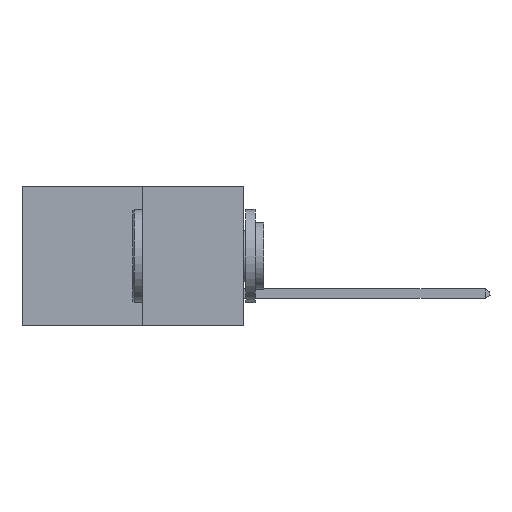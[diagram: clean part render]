
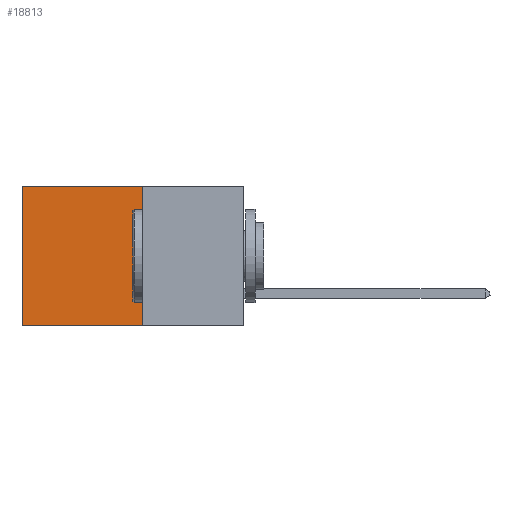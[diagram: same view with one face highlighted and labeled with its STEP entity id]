
A CAD part, left-side view. The second image highlights one B-rep face of the part: STEP entity #18813.
In plain terms, the highlighted planar face has unit normal (-1, 0, 0).
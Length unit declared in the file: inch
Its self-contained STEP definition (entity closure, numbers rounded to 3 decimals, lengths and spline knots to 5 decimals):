
#637 = ORIENTED_EDGE ( 'NONE', *, *, #9866, .T. ) ;
#1463 = LINE ( 'NONE', #20418, #7314 ) ;
#3775 = EDGE_LOOP ( 'NONE', ( #637, #26534, #28555, #9381 ) ) ;
#4281 = LINE ( 'NONE', #24166, #23272 ) ;
#5421 = CARTESIAN_POINT ( 'NONE',  ( 0.277, 0.59, -0.37 ) ) ;
#5788 = EDGE_CURVE ( 'NONE', #28523, #26337, #24713, .T. ) ;
#7314 = VECTOR ( 'NONE', #10616, 39.37008 ) ;
#8589 = CARTESIAN_POINT ( 'NONE',  ( 0.277, 0.27, -0.37 ) ) ;
#8829 = VERTEX_POINT ( 'NONE', #9032 ) ;
#9032 = CARTESIAN_POINT ( 'NONE',  ( 0.277, 0.59, 0. ) ) ;
#9381 = ORIENTED_EDGE ( 'NONE', *, *, #26235, .T. ) ;
#9478 = FACE_OUTER_BOUND ( 'NONE', #3775, .T. ) ;
#9866 = EDGE_CURVE ( 'NONE', #8829, #26337, #4281, .T. ) ;
#10616 = DIRECTION ( 'NONE',  ( 0., 0., -1. ) ) ;
#11100 = DIRECTION ( 'NONE',  ( 0., 0., -1. ) ) ;
#12107 = VERTEX_POINT ( 'NONE', #15718 ) ;
#15718 = CARTESIAN_POINT ( 'NONE',  ( 0.277, 0.27, 0. ) ) ;
#18398 = PLANE ( 'NONE',  #24129 ) ;
#18813 = ADVANCED_FACE ( 'NONE', ( #9478 ), #18398, .F. ) ;
#19409 = VECTOR ( 'NONE', #27190, 39.37008 ) ;
#20418 = CARTESIAN_POINT ( 'NONE',  ( 0.277, 0.27, -0.37 ) ) ;
#22219 = CARTESIAN_POINT ( 'NONE',  ( 0.277, 0.27, -0.37 ) ) ;
#23272 = VECTOR ( 'NONE', #29095, 39.37008 ) ;
#24129 = AXIS2_PLACEMENT_3D ( 'NONE', #8589, #25901, #11100 ) ;
#24166 = CARTESIAN_POINT ( 'NONE',  ( 0.277, 0.59, -0.37 ) ) ;
#24712 = CARTESIAN_POINT ( 'NONE',  ( 0.277, 0.27, 0. ) ) ;
#24713 = LINE ( 'NONE', #28240, #31982 ) ;
#25901 = DIRECTION ( 'NONE',  ( 1., 0., 0. ) ) ;
#26031 = LINE ( 'NONE', #24712, #19409 ) ;
#26235 = EDGE_CURVE ( 'NONE', #12107, #8829, #26031, .T. ) ;
#26337 = VERTEX_POINT ( 'NONE', #5421 ) ;
#26534 = ORIENTED_EDGE ( 'NONE', *, *, #5788, .F. ) ;
#27190 = DIRECTION ( 'NONE',  ( 0., 1., 0. ) ) ;
#28071 = EDGE_CURVE ( 'NONE', #12107, #28523, #1463, .T. ) ;
#28240 = CARTESIAN_POINT ( 'NONE',  ( 0.277, 0.27, -0.37 ) ) ;
#28523 = VERTEX_POINT ( 'NONE', #22219 ) ;
#28528 = DIRECTION ( 'NONE',  ( 0., 1., 0. ) ) ;
#28555 = ORIENTED_EDGE ( 'NONE', *, *, #28071, .F. ) ;
#29095 = DIRECTION ( 'NONE',  ( 0., 0., -1. ) ) ;
#31982 = VECTOR ( 'NONE', #28528, 39.37008 ) ;
